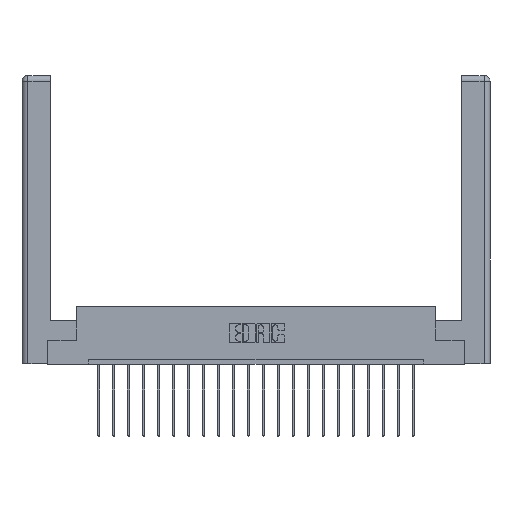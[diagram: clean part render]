
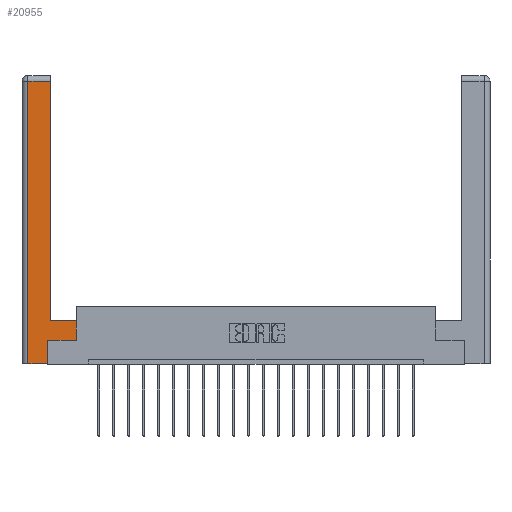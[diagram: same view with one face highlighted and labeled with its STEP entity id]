
A CAD part, top view. The second image highlights one B-rep face of the part: STEP entity #20955.
In plain terms, the highlighted planar face has unit normal (0, 0, 1).
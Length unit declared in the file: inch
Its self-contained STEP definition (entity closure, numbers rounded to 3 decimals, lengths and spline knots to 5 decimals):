
#834 = EDGE_CURVE ( 'NONE', #18179, #14686, #6832, .T. ) ;
#882 = CARTESIAN_POINT ( 'NONE',  ( 0.0615, 0., 0. ) ) ;
#974 = DIRECTION ( 'NONE',  ( -1., 0., 0. ) ) ;
#1090 = DIRECTION ( 'NONE',  ( 0., -1., 0. ) ) ;
#1525 = DIRECTION ( 'NONE',  ( 1., 0., 0. ) ) ;
#1726 = CARTESIAN_POINT ( 'NONE',  ( 0.295, 3., 0. ) ) ;
#2602 = VECTOR ( 'NONE', #5528, 39.37008 ) ;
#2740 = LINE ( 'NONE', #7996, #5056 ) ;
#2811 = CARTESIAN_POINT ( 'NONE',  ( 0.565, 0.245, 0. ) ) ;
#2953 = VECTOR ( 'NONE', #21228, 39.37008 ) ;
#3014 = VERTEX_POINT ( 'NONE', #12452 ) ;
#3642 = CARTESIAN_POINT ( 'NONE',  ( 0.265, 0., 0. ) ) ;
#3994 = CARTESIAN_POINT ( 'NONE',  ( 0.295, 2.94, 0. ) ) ;
#4027 = EDGE_CURVE ( 'NONE', #14686, #11729, #11638, .T. ) ;
#4187 = PLANE ( 'NONE',  #10725 ) ;
#4315 = EDGE_CURVE ( 'NONE', #3014, #9906, #12655, .T. ) ;
#5056 = VECTOR ( 'NONE', #1525, 39.37008 ) ;
#5528 = DIRECTION ( 'NONE',  ( -1., 0., 0. ) ) ;
#5997 = ORIENTED_EDGE ( 'NONE', *, *, #11600, .T. ) ;
#6545 = VECTOR ( 'NONE', #11269, 39.37008 ) ;
#6666 = VECTOR ( 'NONE', #17779, 39.37008 ) ;
#6832 = LINE ( 'NONE', #18787, #17276 ) ;
#7452 = EDGE_CURVE ( 'NONE', #11729, #3014, #14839, .T. ) ;
#7675 = EDGE_CURVE ( 'NONE', #21288, #18121, #15122, .T. ) ;
#7687 = VECTOR ( 'NONE', #10225, 39.37008 ) ;
#7726 = CARTESIAN_POINT ( 'NONE',  ( 0.565, 0.45, 0. ) ) ;
#7996 = CARTESIAN_POINT ( 'NONE',  ( 0.265, 0., 0. ) ) ;
#8385 = CARTESIAN_POINT ( 'NONE',  ( 0.0615, 2.94, 0. ) ) ;
#8881 = LINE ( 'NONE', #16009, #6545 ) ;
#9906 = VERTEX_POINT ( 'NONE', #3994 ) ;
#10225 = DIRECTION ( 'NONE',  ( 0., 1., 0. ) ) ;
#10464 = EDGE_CURVE ( 'NONE', #18121, #15634, #2740, .T. ) ;
#10725 = AXIS2_PLACEMENT_3D ( 'NONE', #15916, #19152, #974 ) ;
#11269 = DIRECTION ( 'NONE',  ( -1., 0., 0. ) ) ;
#11600 = EDGE_CURVE ( 'NONE', #15634, #18179, #14139, .T. ) ;
#11638 = LINE ( 'NONE', #7726, #6666 ) ;
#11665 = CARTESIAN_POINT ( 'NONE',  ( 0.265, 0.245, 0. ) ) ;
#11729 = VERTEX_POINT ( 'NONE', #21515 ) ;
#11866 = ORIENTED_EDGE ( 'NONE', *, *, #20491, .T. ) ;
#12247 = VECTOR ( 'NONE', #1090, 39.37008 ) ;
#12452 = CARTESIAN_POINT ( 'NONE',  ( 0.295, 0.45, 0. ) ) ;
#12655 = LINE ( 'NONE', #1726, #7687 ) ;
#12672 = ORIENTED_EDGE ( 'NONE', *, *, #4315, .T. ) ;
#14139 = LINE ( 'NONE', #19687, #2953 ) ;
#14686 = VERTEX_POINT ( 'NONE', #2811 ) ;
#14839 = LINE ( 'NONE', #20700, #2602 ) ;
#15122 = LINE ( 'NONE', #882, #12247 ) ;
#15262 = ORIENTED_EDGE ( 'NONE', *, *, #10464, .T. ) ;
#15306 = ORIENTED_EDGE ( 'NONE', *, *, #834, .T. ) ;
#15530 = DIRECTION ( 'NONE',  ( 1., 0., 0. ) ) ;
#15634 = VERTEX_POINT ( 'NONE', #3642 ) ;
#15916 = CARTESIAN_POINT ( 'NONE',  ( 0., 0., 0. ) ) ;
#15930 = ORIENTED_EDGE ( 'NONE', *, *, #7675, .T. ) ;
#16009 = CARTESIAN_POINT ( 'NONE',  ( 0.0615, 2.94, 0. ) ) ;
#16449 = FACE_OUTER_BOUND ( 'NONE', #17877, .T. ) ;
#16975 = ORIENTED_EDGE ( 'NONE', *, *, #4027, .T. ) ;
#17276 = VECTOR ( 'NONE', #15530, 39.37008 ) ;
#17779 = DIRECTION ( 'NONE',  ( 0., 1., 0. ) ) ;
#17877 = EDGE_LOOP ( 'NONE', ( #12672, #11866, #15930, #15262, #5997, #15306, #16975, #20885 ) ) ;
#18121 = VERTEX_POINT ( 'NONE', #19600 ) ;
#18179 = VERTEX_POINT ( 'NONE', #11665 ) ;
#18787 = CARTESIAN_POINT ( 'NONE',  ( 0.565, 0.245, 0. ) ) ;
#19152 = DIRECTION ( 'NONE',  ( 0., 0., -1. ) ) ;
#19600 = CARTESIAN_POINT ( 'NONE',  ( 0.0615, 0., 0. ) ) ;
#19687 = CARTESIAN_POINT ( 'NONE',  ( 0.265, 0.245, 0. ) ) ;
#20491 = EDGE_CURVE ( 'NONE', #9906, #21288, #8881, .T. ) ;
#20700 = CARTESIAN_POINT ( 'NONE',  ( 0.295, 0.45, 0. ) ) ;
#20885 = ORIENTED_EDGE ( 'NONE', *, *, #7452, .T. ) ;
#20955 = ADVANCED_FACE ( 'NONE', ( #16449 ), #4187, .F. ) ;
#21228 = DIRECTION ( 'NONE',  ( 0., 1., 0. ) ) ;
#21288 = VERTEX_POINT ( 'NONE', #8385 ) ;
#21515 = CARTESIAN_POINT ( 'NONE',  ( 0.565, 0.45, 0. ) ) ;
